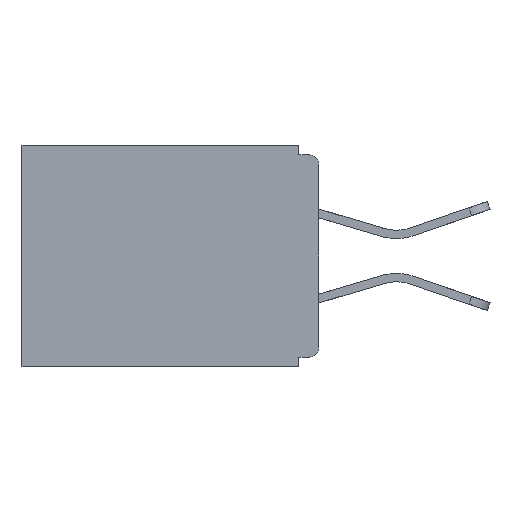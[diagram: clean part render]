
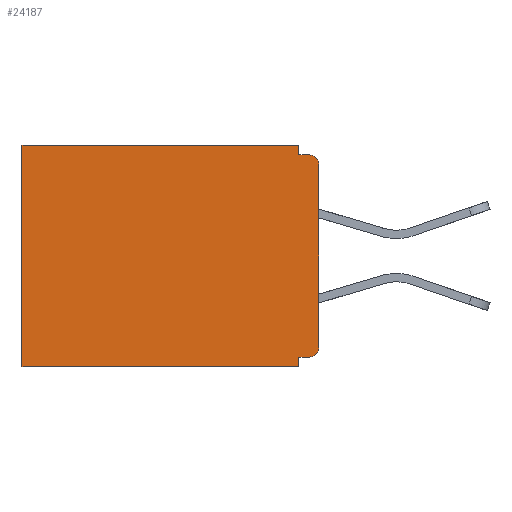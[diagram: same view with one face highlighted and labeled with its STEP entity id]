
A CAD part, left-side view. The second image highlights one B-rep face of the part: STEP entity #24187.
In plain terms, the highlighted planar face has unit normal (-1, 0, 0).
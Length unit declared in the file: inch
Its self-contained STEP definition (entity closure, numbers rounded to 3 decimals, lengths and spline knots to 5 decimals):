
#94 = CARTESIAN_POINT ( 'NONE',  ( 0.298, 0., 0. ) ) ;
#821 = ORIENTED_EDGE ( 'NONE', *, *, #11865, .T. ) ;
#1081 = CARTESIAN_POINT ( 'NONE',  ( 0.298, 0., -0.343 ) ) ;
#1440 = DIRECTION ( 'NONE',  ( 0., 0., -1. ) ) ;
#1446 = AXIS2_PLACEMENT_3D ( 'NONE', #6470, #22892, #25265 ) ;
#1627 = LINE ( 'NONE', #24829, #22183 ) ;
#2270 = CARTESIAN_POINT ( 'NONE',  ( 0.298, 0.031, -0.343 ) ) ;
#2471 = DIRECTION ( 'NONE',  ( 0., 0., -1. ) ) ;
#3191 = LINE ( 'NONE', #1081, #5772 ) ;
#3631 = VECTOR ( 'NONE', #16130, 39.37008 ) ;
#3975 = CARTESIAN_POINT ( 'NONE',  ( 0.298, 0.031, -0.328 ) ) ;
#4055 = ORIENTED_EDGE ( 'NONE', *, *, #29159, .F. ) ;
#4197 = PLANE ( 'NONE',  #1446 ) ;
#4365 = EDGE_CURVE ( 'NONE', #19170, #23951, #1627, .T. ) ;
#4808 = ORIENTED_EDGE ( 'NONE', *, *, #18544, .T. ) ;
#5228 = CARTESIAN_POINT ( 'NONE',  ( 0.298, 0., -0.03 ) ) ;
#5320 = DIRECTION ( 'NONE',  ( 0., 0., -1. ) ) ;
#5539 = CARTESIAN_POINT ( 'NONE',  ( 0.298, 0.015, -0.015 ) ) ;
#5586 = ORIENTED_EDGE ( 'NONE', *, *, #4365, .F. ) ;
#5772 = VECTOR ( 'NONE', #22120, 39.37008 ) ;
#5848 = FACE_OUTER_BOUND ( 'NONE', #10173, .T. ) ;
#6094 = VECTOR ( 'NONE', #2471, 39.37008 ) ;
#6198 = VERTEX_POINT ( 'NONE', #5228 ) ;
#6470 = CARTESIAN_POINT ( 'NONE',  ( 0.298, 0., 0. ) ) ;
#7026 = DIRECTION ( 'NONE',  ( -1., 0., 0. ) ) ;
#7512 = CARTESIAN_POINT ( 'NONE',  ( 0.298, 0.015, -0.313 ) ) ;
#7536 = VERTEX_POINT ( 'NONE', #21594 ) ;
#8051 = CARTESIAN_POINT ( 'NONE',  ( 0.298, 0.031, -0.343 ) ) ;
#8572 = CARTESIAN_POINT ( 'NONE',  ( 0.298, 0.46, 0. ) ) ;
#8725 = EDGE_CURVE ( 'NONE', #9959, #14237, #3191, .T. ) ;
#9022 = LINE ( 'NONE', #20386, #18550 ) ;
#9358 = VERTEX_POINT ( 'NONE', #23999 ) ;
#9407 = VECTOR ( 'NONE', #28132, 39.37008 ) ;
#9692 = CARTESIAN_POINT ( 'NONE',  ( 0.298, 0.031, -0.015 ) ) ;
#9959 = VERTEX_POINT ( 'NONE', #2270 ) ;
#10003 = EDGE_CURVE ( 'NONE', #6198, #7536, #29260, .T. ) ;
#10173 = EDGE_LOOP ( 'NONE', ( #16904, #5586, #4055, #821, #4808, #19187, #14915, #18113, #23316, #18810 ) ) ;
#10509 = EDGE_CURVE ( 'NONE', #9358, #29232, #9022, .T. ) ;
#10726 = EDGE_CURVE ( 'NONE', #29232, #9959, #29934, .T. ) ;
#10776 = DIRECTION ( 'NONE',  ( 0., -1., 0. ) ) ;
#11114 = CARTESIAN_POINT ( 'NONE',  ( 0.298, 0.031, 0. ) ) ;
#11190 = VERTEX_POINT ( 'NONE', #16789 ) ;
#11865 = EDGE_CURVE ( 'NONE', #23989, #11190, #24021, .T. ) ;
#12106 = CARTESIAN_POINT ( 'NONE',  ( 0.298, 0.46, -0.343 ) ) ;
#12769 = CIRCLE ( 'NONE', #30172, 0.015 ) ;
#14237 = VERTEX_POINT ( 'NONE', #12106 ) ;
#14474 = VECTOR ( 'NONE', #1440, 39.37008 ) ;
#14476 = AXIS2_PLACEMENT_3D ( 'NONE', #18536, #7026, #25522 ) ;
#14915 = ORIENTED_EDGE ( 'NONE', *, *, #10726, .F. ) ;
#16130 = DIRECTION ( 'NONE',  ( 0., 0., -1. ) ) ;
#16789 = CARTESIAN_POINT ( 'NONE',  ( 0.298, 0.46, 0. ) ) ;
#16904 = ORIENTED_EDGE ( 'NONE', *, *, #16945, .T. ) ;
#16945 = EDGE_CURVE ( 'NONE', #6198, #23951, #20888, .T. ) ;
#17280 = LINE ( 'NONE', #27618, #3631 ) ;
#18113 = ORIENTED_EDGE ( 'NONE', *, *, #10509, .F. ) ;
#18228 = LINE ( 'NONE', #8572, #9407 ) ;
#18270 = DIRECTION ( 'NONE',  ( 0., 1., 0. ) ) ;
#18536 = CARTESIAN_POINT ( 'NONE',  ( 0.298, 0.015, -0.03 ) ) ;
#18544 = EDGE_CURVE ( 'NONE', #11190, #14237, #18228, .T. ) ;
#18550 = VECTOR ( 'NONE', #23207, 39.37008 ) ;
#18810 = ORIENTED_EDGE ( 'NONE', *, *, #10003, .F. ) ;
#19170 = VERTEX_POINT ( 'NONE', #9692 ) ;
#19187 = ORIENTED_EDGE ( 'NONE', *, *, #8725, .F. ) ;
#20386 = CARTESIAN_POINT ( 'NONE',  ( 0.298, 0., -0.328 ) ) ;
#20888 = CIRCLE ( 'NONE', #14476, 0.015 ) ;
#20920 = CARTESIAN_POINT ( 'NONE',  ( 0.298, 0., 0. ) ) ;
#21109 = VECTOR ( 'NONE', #18270, 39.37008 ) ;
#21594 = CARTESIAN_POINT ( 'NONE',  ( 0.298, 0., -0.313 ) ) ;
#22120 = DIRECTION ( 'NONE',  ( 0., 1., 0. ) ) ;
#22183 = VECTOR ( 'NONE', #10776, 39.37008 ) ;
#22892 = DIRECTION ( 'NONE',  ( 1., 0., 0. ) ) ;
#23207 = DIRECTION ( 'NONE',  ( 0., 1., 0. ) ) ;
#23316 = ORIENTED_EDGE ( 'NONE', *, *, #30241, .T. ) ;
#23951 = VERTEX_POINT ( 'NONE', #5539 ) ;
#23989 = VERTEX_POINT ( 'NONE', #11114 ) ;
#23999 = CARTESIAN_POINT ( 'NONE',  ( 0.298, 0.015, -0.328 ) ) ;
#24021 = LINE ( 'NONE', #20920, #21109 ) ;
#24187 = ADVANCED_FACE ( 'NONE', ( #5848 ), #4197, .F. ) ;
#24829 = CARTESIAN_POINT ( 'NONE',  ( 0.298, 0., -0.015 ) ) ;
#25265 = DIRECTION ( 'NONE',  ( 0., 0., -1. ) ) ;
#25522 = DIRECTION ( 'NONE',  ( 0., 0., -1. ) ) ;
#27618 = CARTESIAN_POINT ( 'NONE',  ( 0.298, 0.031, -0.343 ) ) ;
#28132 = DIRECTION ( 'NONE',  ( 0., 0., -1. ) ) ;
#28542 = DIRECTION ( 'NONE',  ( -1., 0., 0. ) ) ;
#29159 = EDGE_CURVE ( 'NONE', #23989, #19170, #17280, .T. ) ;
#29232 = VERTEX_POINT ( 'NONE', #3975 ) ;
#29260 = LINE ( 'NONE', #94, #6094 ) ;
#29934 = LINE ( 'NONE', #8051, #14474 ) ;
#30172 = AXIS2_PLACEMENT_3D ( 'NONE', #7512, #28542, #5320 ) ;
#30241 = EDGE_CURVE ( 'NONE', #9358, #7536, #12769, .T. ) ;
